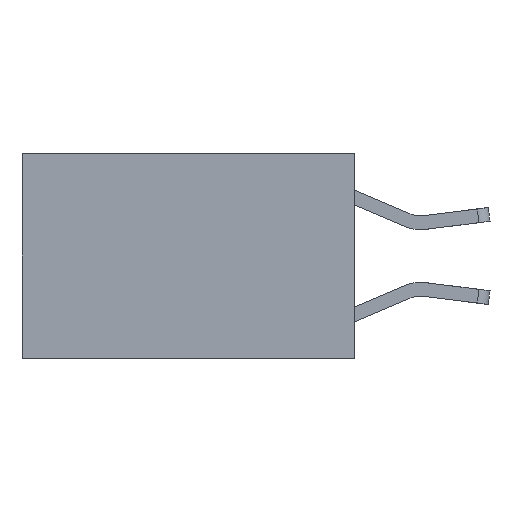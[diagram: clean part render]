
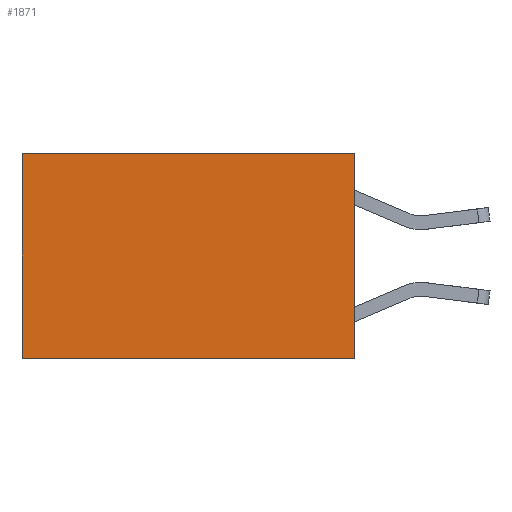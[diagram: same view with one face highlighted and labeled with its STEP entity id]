
A CAD part, left-side view. The second image highlights one B-rep face of the part: STEP entity #1871.
In plain terms, the highlighted planar face has unit normal (-1, 0, 0).
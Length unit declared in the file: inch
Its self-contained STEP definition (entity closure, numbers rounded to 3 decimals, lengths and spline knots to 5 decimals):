
#90 = CARTESIAN_POINT ( 'NONE',  ( 0.2625, 0., 0. ) ) ;
#182 = CARTESIAN_POINT ( 'NONE',  ( 0.2625, 0.6, 0. ) ) ;
#247 = CARTESIAN_POINT ( 'NONE',  ( 0.2625, 0., -0.37 ) ) ;
#367 = FACE_OUTER_BOUND ( 'NONE', #4478, .T. ) ;
#527 = VECTOR ( 'NONE', #6470, 39.37008 ) ;
#1871 = ADVANCED_FACE ( 'NONE', ( #367 ), #9147, .F. ) ;
#2030 = ORIENTED_EDGE ( 'NONE', *, *, #5042, .F. ) ;
#2158 = EDGE_CURVE ( 'NONE', #6035, #8301, #2251, .T. ) ;
#2251 = LINE ( 'NONE', #182, #5519 ) ;
#2972 = DIRECTION ( 'NONE',  ( 1., 0., 0. ) ) ;
#3433 = EDGE_CURVE ( 'NONE', #8342, #8305, #8492, .T. ) ;
#3728 = ORIENTED_EDGE ( 'NONE', *, *, #3433, .F. ) ;
#3934 = ORIENTED_EDGE ( 'NONE', *, *, #5046, .T. ) ;
#4412 = CARTESIAN_POINT ( 'NONE',  ( 0.2625, 0., 0. ) ) ;
#4478 = EDGE_LOOP ( 'NONE', ( #5315, #2030, #3728, #3934 ) ) ;
#5042 = EDGE_CURVE ( 'NONE', #8305, #8301, #8348, .T. ) ;
#5046 = EDGE_CURVE ( 'NONE', #8342, #6035, #8782, .T. ) ;
#5108 = DIRECTION ( 'NONE',  ( 0., 1., 0. ) ) ;
#5212 = DIRECTION ( 'NONE',  ( 0., 0., -1. ) ) ;
#5271 = CARTESIAN_POINT ( 'NONE',  ( 0.2625, 0.6, -0.37 ) ) ;
#5315 = ORIENTED_EDGE ( 'NONE', *, *, #2158, .T. ) ;
#5519 = VECTOR ( 'NONE', #5212, 39.37008 ) ;
#5798 = AXIS2_PLACEMENT_3D ( 'NONE', #8138, #2972, #6665 ) ;
#5971 = CARTESIAN_POINT ( 'NONE',  ( 0.2625, 0., 0. ) ) ;
#6035 = VERTEX_POINT ( 'NONE', #8049 ) ;
#6202 = VECTOR ( 'NONE', #5108, 39.37008 ) ;
#6470 = DIRECTION ( 'NONE',  ( 0., 1., 0. ) ) ;
#6491 = DIRECTION ( 'NONE',  ( 0., 0., -1. ) ) ;
#6665 = DIRECTION ( 'NONE',  ( 0., 0., -1. ) ) ;
#8049 = CARTESIAN_POINT ( 'NONE',  ( 0.2625, 0.6, 0. ) ) ;
#8072 = VECTOR ( 'NONE', #6491, 39.37008 ) ;
#8138 = CARTESIAN_POINT ( 'NONE',  ( 0.2625, 0., 0. ) ) ;
#8301 = VERTEX_POINT ( 'NONE', #5271 ) ;
#8305 = VERTEX_POINT ( 'NONE', #247 ) ;
#8342 = VERTEX_POINT ( 'NONE', #5971 ) ;
#8348 = LINE ( 'NONE', #8619, #6202 ) ;
#8492 = LINE ( 'NONE', #90, #8072 ) ;
#8619 = CARTESIAN_POINT ( 'NONE',  ( 0.2625, 0., -0.37 ) ) ;
#8782 = LINE ( 'NONE', #4412, #527 ) ;
#9147 = PLANE ( 'NONE',  #5798 ) ;
